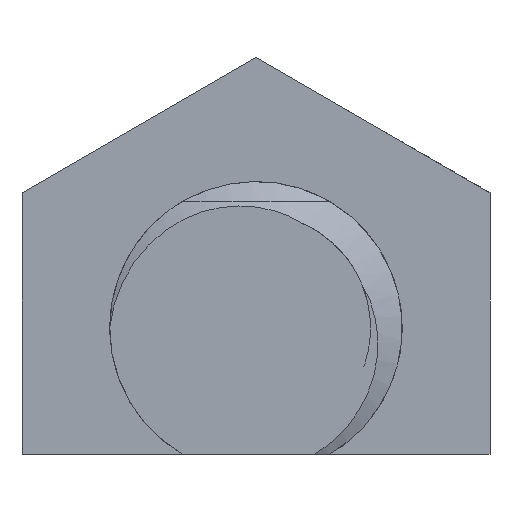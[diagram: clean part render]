
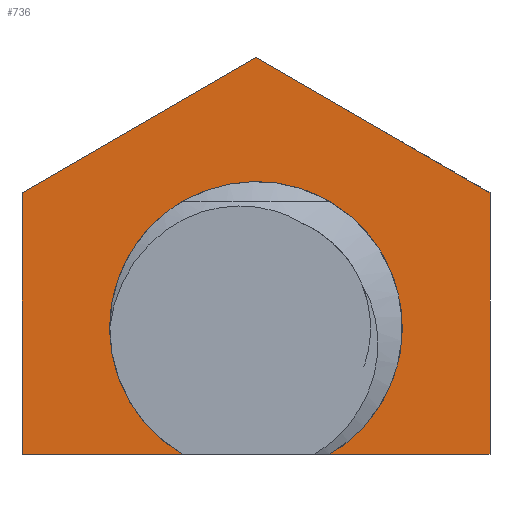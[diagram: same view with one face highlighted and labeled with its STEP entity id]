
A CAD part, left-side view. The second image highlights one B-rep face of the part: STEP entity #736.
In plain terms, the highlighted planar face has unit normal (-1, 0, 0).
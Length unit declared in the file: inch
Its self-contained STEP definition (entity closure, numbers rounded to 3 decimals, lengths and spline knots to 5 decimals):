
#8 = VECTOR ( 'NONE', #2348, 39.37008 ) ;
#68 = VERTEX_POINT ( 'NONE', #1726 ) ;
#224 = EDGE_CURVE ( 'NONE', #895, #1599, #919, .T. ) ;
#229 = LINE ( 'NONE', #855, #1674 ) ;
#230 = DIRECTION ( 'NONE',  ( 0., 0., -1. ) ) ;
#248 = CARTESIAN_POINT ( 'NONE',  ( 0.4425, -0.81272, 0.22357 ) ) ;
#269 = AXIS2_PLACEMENT_3D ( 'NONE', #1547, #1347, #230 ) ;
#291 = LINE ( 'NONE', #1018, #8 ) ;
#448 = VECTOR ( 'NONE', #2250, 39.37008 ) ;
#462 = EDGE_CURVE ( 'NONE', #584, #618, #291, .T. ) ;
#584 = VERTEX_POINT ( 'NONE', #1848 ) ;
#618 = VERTEX_POINT ( 'NONE', #2448 ) ;
#629 = CARTESIAN_POINT ( 'NONE',  ( 0.4425, -0.61272, 0. ) ) ;
#650 = VERTEX_POINT ( 'NONE', #1884 ) ;
#736 = ADVANCED_FACE ( 'NONE', ( #1895 ), #1170, .F. ) ;
#743 = CARTESIAN_POINT ( 'NONE',  ( 0.4425, -0.61272, 0. ) ) ;
#757 = VECTOR ( 'NONE', #1948, 39.37008 ) ;
#777 = DIRECTION ( 'NONE',  ( 0., 0., -1. ) ) ;
#794 = DIRECTION ( 'NONE',  ( -1., 0., 0. ) ) ;
#797 = VECTOR ( 'NONE', #1002, 39.37008 ) ;
#799 = DIRECTION ( 'NONE',  ( 0., 0.866, 0.5 ) ) ;
#855 = CARTESIAN_POINT ( 'NONE',  ( 0.4425, -0.41272, -0.00737 ) ) ;
#895 = VERTEX_POINT ( 'NONE', #1764 ) ;
#898 = DIRECTION ( 'NONE',  ( 0., 0., -1. ) ) ;
#919 = LINE ( 'NONE', #248, #797 ) ;
#1002 = DIRECTION ( 'NONE',  ( 0., 0., 1. ) ) ;
#1018 = CARTESIAN_POINT ( 'NONE',  ( 0.4425, -0.41272, 0.22357 ) ) ;
#1091 = ORIENTED_EDGE ( 'NONE', *, *, #462, .T. ) ;
#1170 = PLANE ( 'NONE',  #269 ) ;
#1196 = CARTESIAN_POINT ( 'NONE',  ( 0.4425, -0.54996, 0. ) ) ;
#1204 = EDGE_CURVE ( 'NONE', #68, #1647, #2082, .T. ) ;
#1294 = ORIENTED_EDGE ( 'NONE', *, *, #2313, .T. ) ;
#1347 = DIRECTION ( 'NONE',  ( 1., 0., 0. ) ) ;
#1388 = EDGE_CURVE ( 'NONE', #68, #895, #1645, .T. ) ;
#1525 = CARTESIAN_POINT ( 'NONE',  ( 0.4425, -0.81272, 0.22357 ) ) ;
#1535 = CARTESIAN_POINT ( 'NONE',  ( 0.4425, -0.61272, 0.1081 ) ) ;
#1547 = CARTESIAN_POINT ( 'NONE',  ( 0.4425, -0.61272, 0.1081 ) ) ;
#1599 = VERTEX_POINT ( 'NONE', #1525 ) ;
#1606 = ORIENTED_EDGE ( 'NONE', *, *, #224, .T. ) ;
#1624 = EDGE_CURVE ( 'NONE', #1599, #584, #2177, .T. ) ;
#1645 = LINE ( 'NONE', #629, #757 ) ;
#1647 = VERTEX_POINT ( 'NONE', #1196 ) ;
#1674 = VECTOR ( 'NONE', #898, 39.37008 ) ;
#1696 = ORIENTED_EDGE ( 'NONE', *, *, #1204, .F. ) ;
#1701 = EDGE_LOOP ( 'NONE', ( #1892, #1294, #1696, #1814, #1606, #2414, #1091 ) ) ;
#1715 = AXIS2_PLACEMENT_3D ( 'NONE', #1535, #794, #777 ) ;
#1726 = CARTESIAN_POINT ( 'NONE',  ( 0.4425, -0.67549, 0. ) ) ;
#1764 = CARTESIAN_POINT ( 'NONE',  ( 0.4425, -0.81272, 0. ) ) ;
#1773 = LINE ( 'NONE', #743, #448 ) ;
#1814 = ORIENTED_EDGE ( 'NONE', *, *, #1388, .T. ) ;
#1848 = CARTESIAN_POINT ( 'NONE',  ( 0.4425, -0.61272, 0.33904 ) ) ;
#1884 = CARTESIAN_POINT ( 'NONE',  ( 0.4425, -0.41272, 0. ) ) ;
#1892 = ORIENTED_EDGE ( 'NONE', *, *, #2208, .T. ) ;
#1895 = FACE_OUTER_BOUND ( 'NONE', #1701, .T. ) ;
#1918 = CARTESIAN_POINT ( 'NONE',  ( 0.4425, -0.61272, 0.33904 ) ) ;
#1948 = DIRECTION ( 'NONE',  ( 0., -1., 0. ) ) ;
#2082 = CIRCLE ( 'NONE', #1715, 0.125 ) ;
#2177 = LINE ( 'NONE', #1918, #2232 ) ;
#2208 = EDGE_CURVE ( 'NONE', #618, #650, #229, .T. ) ;
#2232 = VECTOR ( 'NONE', #799, 39.37008 ) ;
#2250 = DIRECTION ( 'NONE',  ( 0., -1., 0. ) ) ;
#2313 = EDGE_CURVE ( 'NONE', #650, #1647, #1773, .T. ) ;
#2348 = DIRECTION ( 'NONE',  ( 0., 0.866, -0.5 ) ) ;
#2414 = ORIENTED_EDGE ( 'NONE', *, *, #1624, .T. ) ;
#2448 = CARTESIAN_POINT ( 'NONE',  ( 0.4425, -0.41272, 0.22357 ) ) ;
